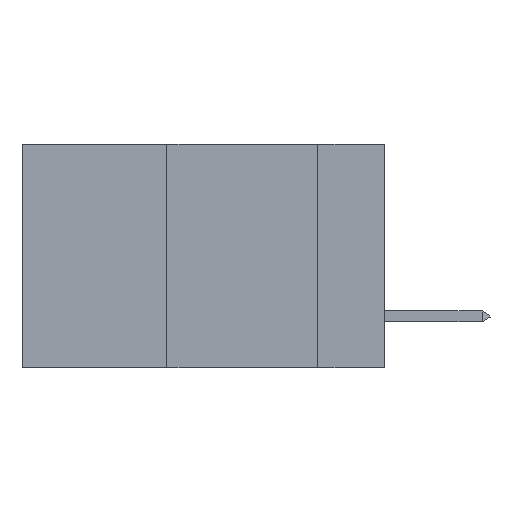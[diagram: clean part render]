
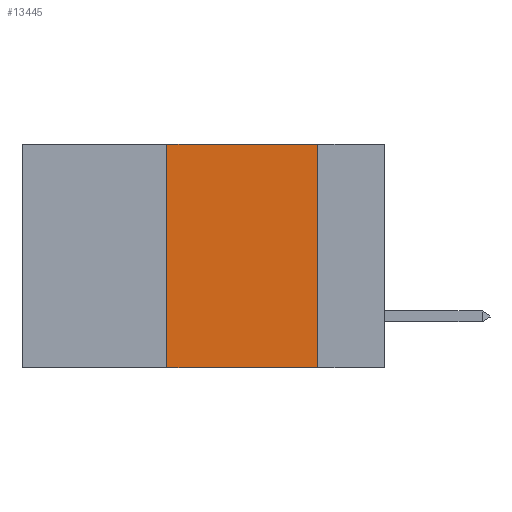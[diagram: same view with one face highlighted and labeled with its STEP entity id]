
A CAD part, left-side view. The second image highlights one B-rep face of the part: STEP entity #13445.
In plain terms, the highlighted planar face has unit normal (-1, 0, 0).
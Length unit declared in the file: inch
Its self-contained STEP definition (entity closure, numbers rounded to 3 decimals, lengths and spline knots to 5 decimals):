
#696 = VERTEX_POINT ( 'NONE', #23374 ) ;
#1814 = DIRECTION ( 'NONE',  ( 0., 0., -1. ) ) ;
#4189 = LINE ( 'NONE', #12823, #28271 ) ;
#7323 = VERTEX_POINT ( 'NONE', #32174 ) ;
#7962 = CARTESIAN_POINT ( 'NONE',  ( 0., 0.36, -0.37 ) ) ;
#10335 = ORIENTED_EDGE ( 'NONE', *, *, #14110, .F. ) ;
#10663 = EDGE_CURVE ( 'NONE', #696, #19219, #22454, .T. ) ;
#12823 = CARTESIAN_POINT ( 'NONE',  ( 0., 0.6, 0. ) ) ;
#12936 = FACE_OUTER_BOUND ( 'NONE', #28734, .T. ) ;
#13445 = ADVANCED_FACE ( 'NONE', ( #12936 ), #39240, .F. ) ;
#14082 = VECTOR ( 'NONE', #21357, 39.37008 ) ;
#14110 = EDGE_CURVE ( 'NONE', #35447, #7323, #22415, .T. ) ;
#16764 = CARTESIAN_POINT ( 'NONE',  ( 0., 0.11, -0.37 ) ) ;
#17010 = EDGE_CURVE ( 'NONE', #35447, #19219, #27585, .T. ) ;
#18019 = DIRECTION ( 'NONE',  ( 0., -1., 0. ) ) ;
#18192 = CARTESIAN_POINT ( 'NONE',  ( 0., 0.36, 0. ) ) ;
#19109 = DIRECTION ( 'NONE',  ( 0., -1., 0. ) ) ;
#19219 = VERTEX_POINT ( 'NONE', #16764 ) ;
#20802 = DIRECTION ( 'NONE',  ( 1., 0., 0. ) ) ;
#21357 = DIRECTION ( 'NONE',  ( 0., 0., 1. ) ) ;
#22114 = ORIENTED_EDGE ( 'NONE', *, *, #10663, .F. ) ;
#22415 = LINE ( 'NONE', #18192, #14082 ) ;
#22454 = LINE ( 'NONE', #35383, #37822 ) ;
#23374 = CARTESIAN_POINT ( 'NONE',  ( 0., 0.11, 0. ) ) ;
#23869 = CARTESIAN_POINT ( 'NONE',  ( 0., 0.6, 0. ) ) ;
#24735 = AXIS2_PLACEMENT_3D ( 'NONE', #23869, #20802, #1814 ) ;
#26625 = VECTOR ( 'NONE', #18019, 39.37008 ) ;
#27016 = ORIENTED_EDGE ( 'NONE', *, *, #17010, .T. ) ;
#27585 = LINE ( 'NONE', #30364, #26625 ) ;
#28271 = VECTOR ( 'NONE', #19109, 39.37008 ) ;
#28734 = EDGE_LOOP ( 'NONE', ( #22114, #32216, #10335, #27016 ) ) ;
#30364 = CARTESIAN_POINT ( 'NONE',  ( 0., 0.6, -0.37 ) ) ;
#32174 = CARTESIAN_POINT ( 'NONE',  ( 0., 0.36, 0. ) ) ;
#32216 = ORIENTED_EDGE ( 'NONE', *, *, #40084, .F. ) ;
#35383 = CARTESIAN_POINT ( 'NONE',  ( 0., 0.11, 0. ) ) ;
#35447 = VERTEX_POINT ( 'NONE', #7962 ) ;
#37822 = VECTOR ( 'NONE', #38486, 39.37008 ) ;
#38486 = DIRECTION ( 'NONE',  ( 0., 0., -1. ) ) ;
#39240 = PLANE ( 'NONE',  #24735 ) ;
#40084 = EDGE_CURVE ( 'NONE', #7323, #696, #4189, .T. ) ;
